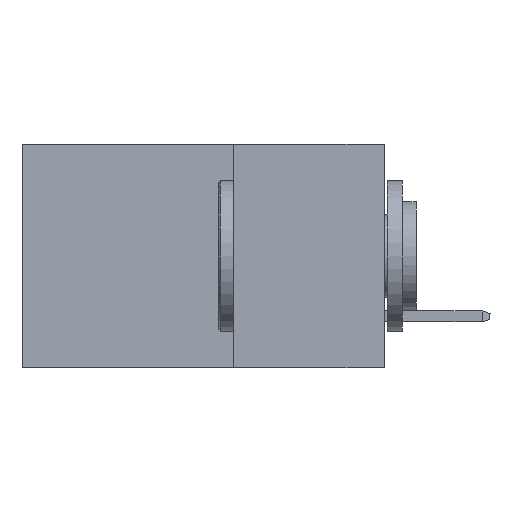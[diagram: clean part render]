
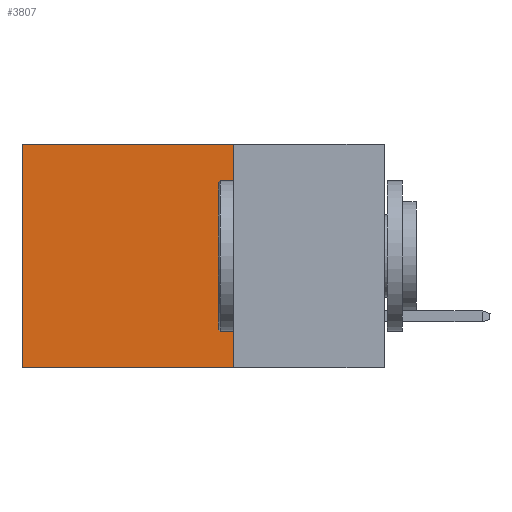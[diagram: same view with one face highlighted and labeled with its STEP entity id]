
A CAD part, left-side view. The second image highlights one B-rep face of the part: STEP entity #3807.
In plain terms, the highlighted planar face has unit normal (-1, 0, 0).
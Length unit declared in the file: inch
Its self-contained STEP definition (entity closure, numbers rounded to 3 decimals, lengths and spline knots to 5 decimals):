
#191 = DIRECTION ( 'NONE',  ( 0., 0., -1. ) ) ;
#267 = DIRECTION ( 'NONE',  ( 0., 1., 0. ) ) ;
#431 = EDGE_CURVE ( 'NONE', #11440, #3950, #2651, .T. ) ;
#1160 = VERTEX_POINT ( 'NONE', #2296 ) ;
#1449 = VERTEX_POINT ( 'NONE', #1798 ) ;
#1515 = CARTESIAN_POINT ( 'NONE',  ( 0.2615, 0.6, -0.37 ) ) ;
#1743 = DIRECTION ( 'NONE',  ( 0., 0., -1. ) ) ;
#1798 = CARTESIAN_POINT ( 'NONE',  ( 0.2615, 0.25, 0. ) ) ;
#2296 = CARTESIAN_POINT ( 'NONE',  ( 0.2615, 0.25, -0.37 ) ) ;
#2651 = LINE ( 'NONE', #4288, #9563 ) ;
#2748 = ORIENTED_EDGE ( 'NONE', *, *, #3446, .T. ) ;
#3170 = CARTESIAN_POINT ( 'NONE',  ( 0.2615, 0.25, -0.37 ) ) ;
#3446 = EDGE_CURVE ( 'NONE', #1449, #11440, #6178, .T. ) ;
#3789 = EDGE_LOOP ( 'NONE', ( #10601, #7757, #9400, #2748 ) ) ;
#3807 = ADVANCED_FACE ( 'NONE', ( #4065 ), #9461, .F. ) ;
#3950 = VERTEX_POINT ( 'NONE', #1515 ) ;
#4065 = FACE_OUTER_BOUND ( 'NONE', #3789, .T. ) ;
#4288 = CARTESIAN_POINT ( 'NONE',  ( 0.2615, 0.6, -0.37 ) ) ;
#4891 = VECTOR ( 'NONE', #267, 39.37008 ) ;
#5045 = CARTESIAN_POINT ( 'NONE',  ( 0.2615, 0.6, 0. ) ) ;
#5404 = AXIS2_PLACEMENT_3D ( 'NONE', #9406, #9579, #191 ) ;
#6178 = LINE ( 'NONE', #6959, #8498 ) ;
#6409 = EDGE_CURVE ( 'NONE', #1160, #3950, #8559, .T. ) ;
#6959 = CARTESIAN_POINT ( 'NONE',  ( 0.2615, 0.25, 0. ) ) ;
#7084 = DIRECTION ( 'NONE',  ( 0., 1., 0. ) ) ;
#7247 = LINE ( 'NONE', #10958, #8983 ) ;
#7757 = ORIENTED_EDGE ( 'NONE', *, *, #6409, .F. ) ;
#8498 = VECTOR ( 'NONE', #7084, 39.37008 ) ;
#8559 = LINE ( 'NONE', #3170, #4891 ) ;
#8983 = VECTOR ( 'NONE', #1743, 39.37008 ) ;
#9400 = ORIENTED_EDGE ( 'NONE', *, *, #10817, .F. ) ;
#9406 = CARTESIAN_POINT ( 'NONE',  ( 0.2615, 0.25, -0.37 ) ) ;
#9461 = PLANE ( 'NONE',  #5404 ) ;
#9563 = VECTOR ( 'NONE', #10769, 39.37008 ) ;
#9579 = DIRECTION ( 'NONE',  ( 1., 0., 0. ) ) ;
#10601 = ORIENTED_EDGE ( 'NONE', *, *, #431, .T. ) ;
#10769 = DIRECTION ( 'NONE',  ( 0., 0., -1. ) ) ;
#10817 = EDGE_CURVE ( 'NONE', #1449, #1160, #7247, .T. ) ;
#10958 = CARTESIAN_POINT ( 'NONE',  ( 0.2615, 0.25, -0.37 ) ) ;
#11440 = VERTEX_POINT ( 'NONE', #5045 ) ;
